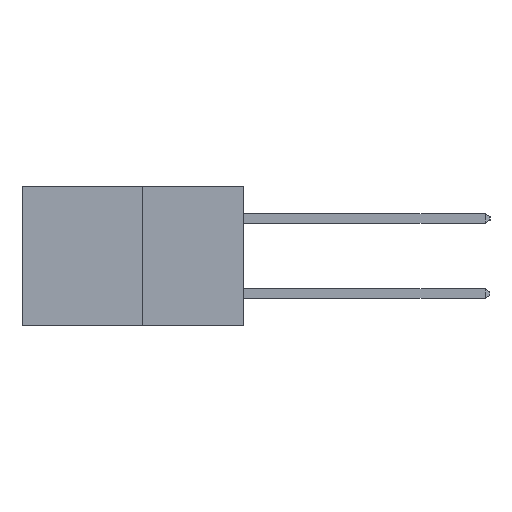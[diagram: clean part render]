
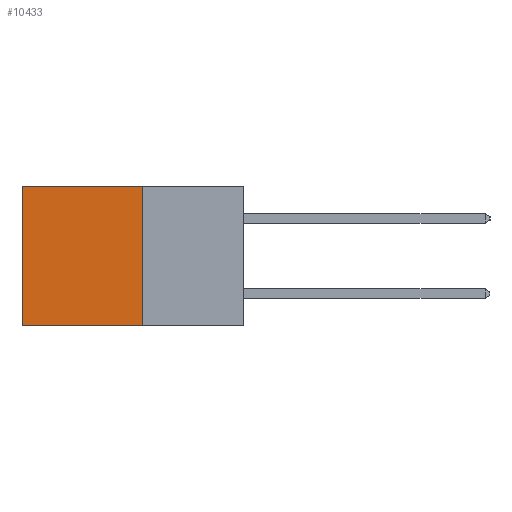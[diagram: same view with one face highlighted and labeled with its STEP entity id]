
A CAD part, left-side view. The second image highlights one B-rep face of the part: STEP entity #10433.
In plain terms, the highlighted planar face has unit normal (-1, 0, 0).
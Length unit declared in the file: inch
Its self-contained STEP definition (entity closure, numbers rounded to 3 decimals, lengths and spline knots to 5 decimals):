
#1329 = DIRECTION ( 'NONE',  ( 0., 0., -1. ) ) ;
#1888 = ORIENTED_EDGE ( 'NONE', *, *, #6709, .T. ) ;
#1981 = EDGE_LOOP ( 'NONE', ( #1888, #11015, #19114, #3456 ) ) ;
#2876 = DIRECTION ( 'NONE',  ( 0., 1., 0. ) ) ;
#3159 = DIRECTION ( 'NONE',  ( 0., 0., -1. ) ) ;
#3456 = ORIENTED_EDGE ( 'NONE', *, *, #13816, .T. ) ;
#3843 = PLANE ( 'NONE',  #9416 ) ;
#4177 = CARTESIAN_POINT ( 'NONE',  ( 0.277, 0.59, 0. ) ) ;
#4421 = CARTESIAN_POINT ( 'NONE',  ( 0.277, 0.27, -0.37 ) ) ;
#4607 = LINE ( 'NONE', #4421, #8478 ) ;
#4874 = CARTESIAN_POINT ( 'NONE',  ( 0.277, 0.59, -0.37 ) ) ;
#4902 = LINE ( 'NONE', #7794, #16451 ) ;
#5194 = VERTEX_POINT ( 'NONE', #4177 ) ;
#5450 = CARTESIAN_POINT ( 'NONE',  ( 0.277, 0.27, -0.37 ) ) ;
#6709 = EDGE_CURVE ( 'NONE', #5194, #16701, #10534, .T. ) ;
#6912 = FACE_OUTER_BOUND ( 'NONE', #1981, .T. ) ;
#7146 = DIRECTION ( 'NONE',  ( 1., 0., 0. ) ) ;
#7794 = CARTESIAN_POINT ( 'NONE',  ( 0.277, 0.27, 0. ) ) ;
#8478 = VECTOR ( 'NONE', #9336, 39.37008 ) ;
#9110 = EDGE_CURVE ( 'NONE', #13889, #16701, #4607, .T. ) ;
#9336 = DIRECTION ( 'NONE',  ( 0., 1., 0. ) ) ;
#9416 = AXIS2_PLACEMENT_3D ( 'NONE', #5450, #7146, #17953 ) ;
#9581 = CARTESIAN_POINT ( 'NONE',  ( 0.277, 0.27, -0.37 ) ) ;
#9952 = CARTESIAN_POINT ( 'NONE',  ( 0.277, 0.59, -0.37 ) ) ;
#9968 = EDGE_CURVE ( 'NONE', #17193, #13889, #18306, .T. ) ;
#10433 = ADVANCED_FACE ( 'NONE', ( #6912 ), #3843, .F. ) ;
#10534 = LINE ( 'NONE', #9952, #14119 ) ;
#11015 = ORIENTED_EDGE ( 'NONE', *, *, #9110, .F. ) ;
#13816 = EDGE_CURVE ( 'NONE', #17193, #5194, #4902, .T. ) ;
#13889 = VERTEX_POINT ( 'NONE', #20226 ) ;
#14119 = VECTOR ( 'NONE', #1329, 39.37008 ) ;
#16451 = VECTOR ( 'NONE', #2876, 39.37008 ) ;
#16701 = VERTEX_POINT ( 'NONE', #4874 ) ;
#17193 = VERTEX_POINT ( 'NONE', #19208 ) ;
#17828 = VECTOR ( 'NONE', #3159, 39.37008 ) ;
#17953 = DIRECTION ( 'NONE',  ( 0., 0., -1. ) ) ;
#18306 = LINE ( 'NONE', #9581, #17828 ) ;
#19114 = ORIENTED_EDGE ( 'NONE', *, *, #9968, .F. ) ;
#19208 = CARTESIAN_POINT ( 'NONE',  ( 0.277, 0.27, 0. ) ) ;
#20226 = CARTESIAN_POINT ( 'NONE',  ( 0.277, 0.27, -0.37 ) ) ;
